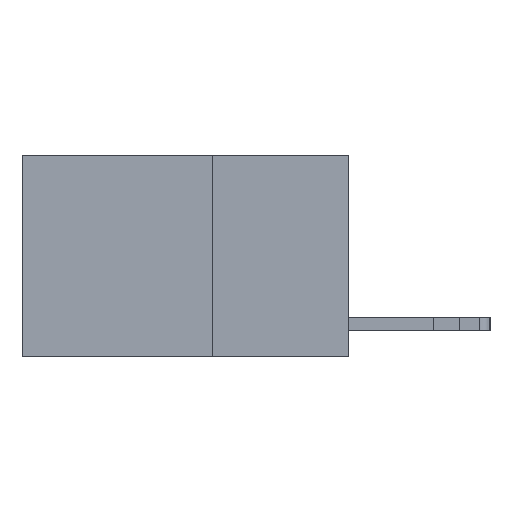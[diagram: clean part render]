
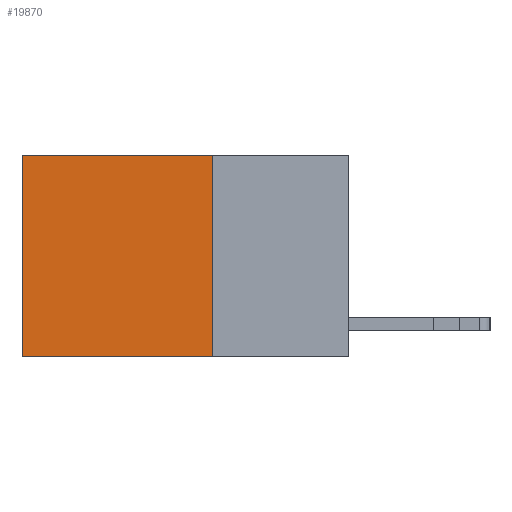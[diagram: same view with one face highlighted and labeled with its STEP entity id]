
A CAD part, left-side view. The second image highlights one B-rep face of the part: STEP entity #19870.
In plain terms, the highlighted planar face has unit normal (-1, 0, 0).
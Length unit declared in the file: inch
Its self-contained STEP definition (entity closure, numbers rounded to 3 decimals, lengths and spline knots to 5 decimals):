
#1633 = VERTEX_POINT ( 'NONE', #6109 ) ;
#2712 = DIRECTION ( 'NONE',  ( 0., 1., 0. ) ) ;
#4807 = CARTESIAN_POINT ( 'NONE',  ( 0.2625, 0.25, -0.37 ) ) ;
#5110 = VECTOR ( 'NONE', #17925, 39.37008 ) ;
#5260 = LINE ( 'NONE', #10838, #12143 ) ;
#5533 = VERTEX_POINT ( 'NONE', #13540 ) ;
#5589 = DIRECTION ( 'NONE',  ( 0., 0., -1. ) ) ;
#5602 = DIRECTION ( 'NONE',  ( 0., 1., 0. ) ) ;
#5875 = AXIS2_PLACEMENT_3D ( 'NONE', #7221, #7339, #5589 ) ;
#5902 = EDGE_CURVE ( 'NONE', #12520, #5533, #16732, .T. ) ;
#6109 = CARTESIAN_POINT ( 'NONE',  ( 0.2625, 0.25, -0.37 ) ) ;
#7221 = CARTESIAN_POINT ( 'NONE',  ( 0.2625, 0.25, 0. ) ) ;
#7339 = DIRECTION ( 'NONE',  ( 1., 0., 0. ) ) ;
#8329 = EDGE_CURVE ( 'NONE', #1633, #5533, #20793, .T. ) ;
#9740 = DIRECTION ( 'NONE',  ( 0., 0., -1. ) ) ;
#9823 = VECTOR ( 'NONE', #9740, 39.37008 ) ;
#9854 = VECTOR ( 'NONE', #2712, 39.37008 ) ;
#10564 = ORIENTED_EDGE ( 'NONE', *, *, #5902, .T. ) ;
#10838 = CARTESIAN_POINT ( 'NONE',  ( 0.2625, 0.25, 0. ) ) ;
#11022 = EDGE_LOOP ( 'NONE', ( #10564, #16188, #11587, #18430 ) ) ;
#11587 = ORIENTED_EDGE ( 'NONE', *, *, #19213, .F. ) ;
#12143 = VECTOR ( 'NONE', #5602, 39.37008 ) ;
#12520 = VERTEX_POINT ( 'NONE', #23097 ) ;
#12798 = CARTESIAN_POINT ( 'NONE',  ( 0.2625, 0.25, 0. ) ) ;
#13540 = CARTESIAN_POINT ( 'NONE',  ( 0.2625, 0.6, -0.37 ) ) ;
#14566 = PLANE ( 'NONE',  #5875 ) ;
#16188 = ORIENTED_EDGE ( 'NONE', *, *, #8329, .F. ) ;
#16718 = EDGE_CURVE ( 'NONE', #17495, #12520, #5260, .T. ) ;
#16732 = LINE ( 'NONE', #18724, #9823 ) ;
#17495 = VERTEX_POINT ( 'NONE', #21815 ) ;
#17925 = DIRECTION ( 'NONE',  ( 0., 0., -1. ) ) ;
#18430 = ORIENTED_EDGE ( 'NONE', *, *, #16718, .T. ) ;
#18724 = CARTESIAN_POINT ( 'NONE',  ( 0.2625, 0.6, 0. ) ) ;
#19213 = EDGE_CURVE ( 'NONE', #17495, #1633, #20988, .T. ) ;
#19870 = ADVANCED_FACE ( 'NONE', ( #21235 ), #14566, .F. ) ;
#20793 = LINE ( 'NONE', #4807, #9854 ) ;
#20988 = LINE ( 'NONE', #12798, #5110 ) ;
#21235 = FACE_OUTER_BOUND ( 'NONE', #11022, .T. ) ;
#21815 = CARTESIAN_POINT ( 'NONE',  ( 0.2625, 0.25, 0. ) ) ;
#23097 = CARTESIAN_POINT ( 'NONE',  ( 0.2625, 0.6, 0. ) ) ;
